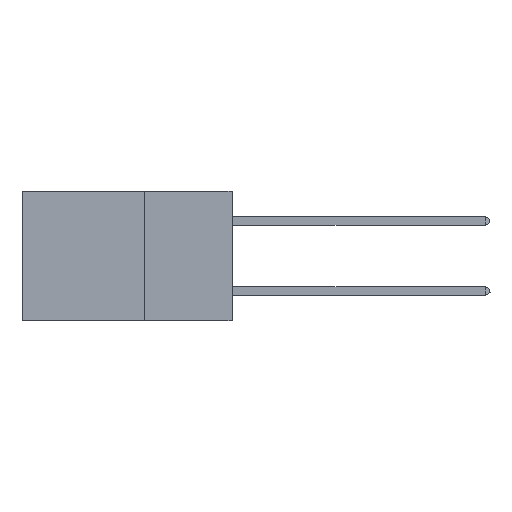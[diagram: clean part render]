
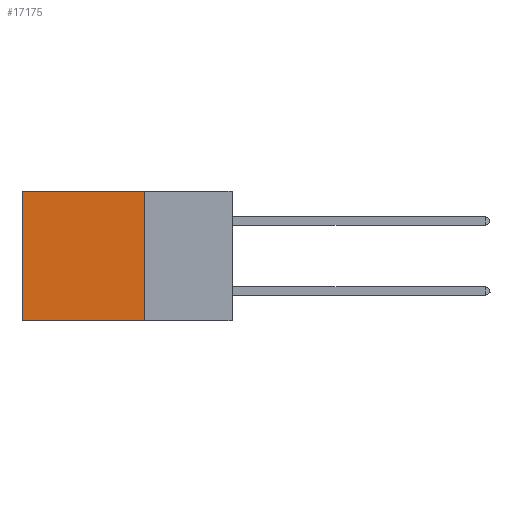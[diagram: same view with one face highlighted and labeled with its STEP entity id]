
A CAD part, left-side view. The second image highlights one B-rep face of the part: STEP entity #17175.
In plain terms, the highlighted planar face has unit normal (-1, 0, 0).
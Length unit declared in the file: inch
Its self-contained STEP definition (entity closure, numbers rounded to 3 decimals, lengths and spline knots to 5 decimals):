
#250 = PLANE ( 'NONE',  #5836 ) ;
#863 = CARTESIAN_POINT ( 'NONE',  ( 0.2875, 0.25, 0. ) ) ;
#2486 = DIRECTION ( 'NONE',  ( 0., 1., 0. ) ) ;
#2622 = CARTESIAN_POINT ( 'NONE',  ( 0.2875, 0.25, 0. ) ) ;
#2982 = CARTESIAN_POINT ( 'NONE',  ( 0.2875, 0.6, 0. ) ) ;
#3637 = EDGE_CURVE ( 'NONE', #24272, #10538, #18455, .T. ) ;
#4044 = FACE_OUTER_BOUND ( 'NONE', #12198, .T. ) ;
#4149 = ORIENTED_EDGE ( 'NONE', *, *, #21261, .F. ) ;
#4448 = LINE ( 'NONE', #863, #12616 ) ;
#5836 = AXIS2_PLACEMENT_3D ( 'NONE', #5962, #9878, #17474 ) ;
#5870 = CARTESIAN_POINT ( 'NONE',  ( 0.2875, 0.25, -0.37 ) ) ;
#5962 = CARTESIAN_POINT ( 'NONE',  ( 0.2875, 0.25, 0. ) ) ;
#6160 = CARTESIAN_POINT ( 'NONE',  ( 0.2875, 0.25, -0.37 ) ) ;
#8665 = DIRECTION ( 'NONE',  ( 0., 0., -1. ) ) ;
#9380 = VERTEX_POINT ( 'NONE', #11640 ) ;
#9878 = DIRECTION ( 'NONE',  ( 1., 0., 0. ) ) ;
#10538 = VERTEX_POINT ( 'NONE', #20694 ) ;
#11640 = CARTESIAN_POINT ( 'NONE',  ( 0.2875, 0.6, -0.37 ) ) ;
#12122 = CARTESIAN_POINT ( 'NONE',  ( 0.2875, 0.25, 0. ) ) ;
#12198 = EDGE_LOOP ( 'NONE', ( #18087, #12977, #4149, #20320 ) ) ;
#12616 = VECTOR ( 'NONE', #13020, 39.37008 ) ;
#12977 = ORIENTED_EDGE ( 'NONE', *, *, #22948, .F. ) ;
#13020 = DIRECTION ( 'NONE',  ( 0., 0., -1. ) ) ;
#15279 = VECTOR ( 'NONE', #8665, 39.37008 ) ;
#15418 = VECTOR ( 'NONE', #19426, 39.37008 ) ;
#16650 = VECTOR ( 'NONE', #2486, 39.37008 ) ;
#17175 = ADVANCED_FACE ( 'NONE', ( #4044 ), #250, .F. ) ;
#17474 = DIRECTION ( 'NONE',  ( 0., 0., -1. ) ) ;
#18087 = ORIENTED_EDGE ( 'NONE', *, *, #22568, .T. ) ;
#18455 = LINE ( 'NONE', #12122, #16650 ) ;
#19426 = DIRECTION ( 'NONE',  ( 0., 1., 0. ) ) ;
#19828 = LINE ( 'NONE', #2982, #15279 ) ;
#20320 = ORIENTED_EDGE ( 'NONE', *, *, #3637, .T. ) ;
#20694 = CARTESIAN_POINT ( 'NONE',  ( 0.2875, 0.6, 0. ) ) ;
#21261 = EDGE_CURVE ( 'NONE', #24272, #23533, #4448, .T. ) ;
#21528 = LINE ( 'NONE', #5870, #15418 ) ;
#22568 = EDGE_CURVE ( 'NONE', #10538, #9380, #19828, .T. ) ;
#22948 = EDGE_CURVE ( 'NONE', #23533, #9380, #21528, .T. ) ;
#23533 = VERTEX_POINT ( 'NONE', #6160 ) ;
#24272 = VERTEX_POINT ( 'NONE', #2622 ) ;
